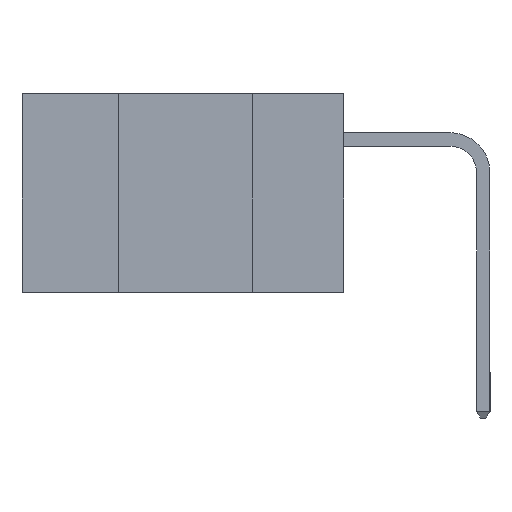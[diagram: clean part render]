
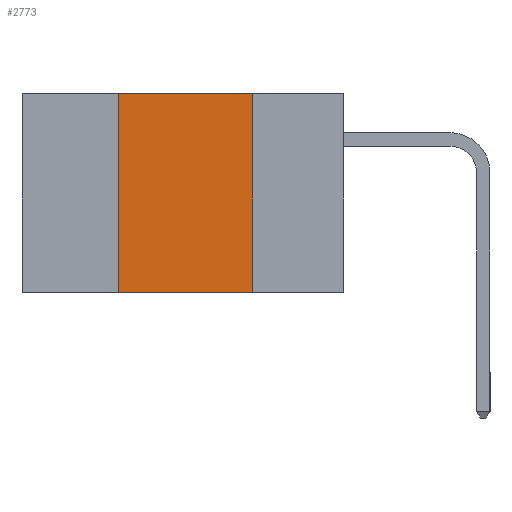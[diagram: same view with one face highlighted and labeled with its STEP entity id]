
A CAD part, left-side view. The second image highlights one B-rep face of the part: STEP entity #2773.
In plain terms, the highlighted planar face has unit normal (-1, 0, 0).
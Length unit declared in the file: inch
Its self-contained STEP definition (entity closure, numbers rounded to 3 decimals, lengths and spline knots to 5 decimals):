
#33 = DIRECTION ( 'NONE',  ( 0., -1., 0. ) ) ;
#187 = CARTESIAN_POINT ( 'NONE',  ( 0., 0.17, -0.37 ) ) ;
#582 = FACE_OUTER_BOUND ( 'NONE', #9839, .T. ) ;
#1122 = LINE ( 'NONE', #4656, #15017 ) ;
#2120 = ORIENTED_EDGE ( 'NONE', *, *, #15674, .F. ) ;
#2349 = LINE ( 'NONE', #8451, #5673 ) ;
#2773 = ADVANCED_FACE ( 'NONE', ( #582 ), #10460, .F. ) ;
#2861 = ORIENTED_EDGE ( 'NONE', *, *, #10436, .F. ) ;
#2906 = DIRECTION ( 'NONE',  ( 0., 0., -1. ) ) ;
#3323 = DIRECTION ( 'NONE',  ( 0., 0., 1. ) ) ;
#3407 = VERTEX_POINT ( 'NONE', #10829 ) ;
#4198 = DIRECTION ( 'NONE',  ( 1., 0., 0. ) ) ;
#4524 = CARTESIAN_POINT ( 'NONE',  ( 0., 0.17, 0. ) ) ;
#4656 = CARTESIAN_POINT ( 'NONE',  ( 0., 0.17, -0.37 ) ) ;
#5494 = CARTESIAN_POINT ( 'NONE',  ( 0., 0.42, -0.37 ) ) ;
#5673 = VECTOR ( 'NONE', #33, 39.37008 ) ;
#5794 = DIRECTION ( 'NONE',  ( 0., 0., -1. ) ) ;
#6521 = DIRECTION ( 'NONE',  ( 0., -1., 0. ) ) ;
#6625 = CARTESIAN_POINT ( 'NONE',  ( 0., 0.6, 0. ) ) ;
#6752 = CARTESIAN_POINT ( 'NONE',  ( 0., 0.6, -0.37 ) ) ;
#8448 = VERTEX_POINT ( 'NONE', #11105 ) ;
#8451 = CARTESIAN_POINT ( 'NONE',  ( 0., 0.6, 0. ) ) ;
#9839 = EDGE_LOOP ( 'NONE', ( #2120, #2861, #13866, #14755 ) ) ;
#9974 = VERTEX_POINT ( 'NONE', #4524 ) ;
#9994 = EDGE_CURVE ( 'NONE', #8448, #3407, #14276, .T. ) ;
#10436 = EDGE_CURVE ( 'NONE', #3407, #9974, #2349, .T. ) ;
#10460 = PLANE ( 'NONE',  #11638 ) ;
#10551 = VERTEX_POINT ( 'NONE', #187 ) ;
#10829 = CARTESIAN_POINT ( 'NONE',  ( 0., 0.42, 0. ) ) ;
#11105 = CARTESIAN_POINT ( 'NONE',  ( 0., 0.42, -0.37 ) ) ;
#11638 = AXIS2_PLACEMENT_3D ( 'NONE', #6625, #4198, #2906 ) ;
#11706 = VECTOR ( 'NONE', #3323, 39.37008 ) ;
#12817 = LINE ( 'NONE', #6752, #15773 ) ;
#13866 = ORIENTED_EDGE ( 'NONE', *, *, #9994, .F. ) ;
#14276 = LINE ( 'NONE', #5494, #11706 ) ;
#14755 = ORIENTED_EDGE ( 'NONE', *, *, #14974, .T. ) ;
#14974 = EDGE_CURVE ( 'NONE', #8448, #10551, #12817, .T. ) ;
#15017 = VECTOR ( 'NONE', #5794, 39.37008 ) ;
#15674 = EDGE_CURVE ( 'NONE', #9974, #10551, #1122, .T. ) ;
#15773 = VECTOR ( 'NONE', #6521, 39.37008 ) ;
